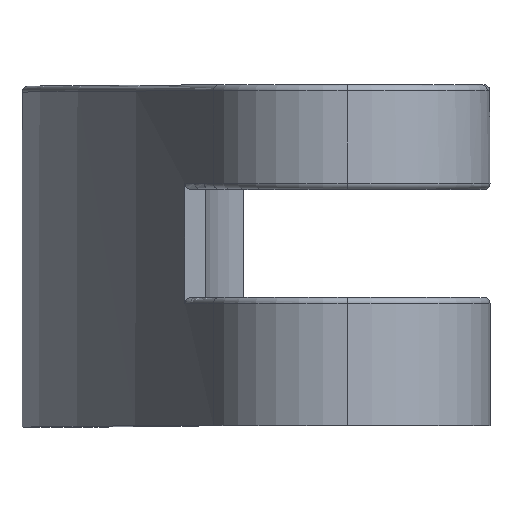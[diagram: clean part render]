
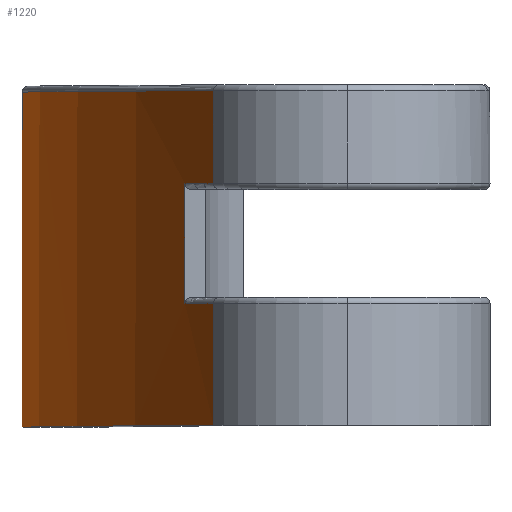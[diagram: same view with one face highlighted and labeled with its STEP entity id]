
A CAD part, top view. The second image highlights one B-rep face of the part: STEP entity #1220.
In plain terms, the highlighted cylindrical face has radius 180.483 mm (diameter 360.965 mm), a partial arc.
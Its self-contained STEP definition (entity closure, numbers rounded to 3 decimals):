
#23 = ORIENTED_EDGE ( 'NONE', *, *, #2267, .T. ) ;
#25 = DIRECTION ( 'NONE',  ( 0., 0., 1. ) ) ;
#28 = CIRCLE ( 'NONE', #1642, 180.483 ) ;
#90 = CARTESIAN_POINT ( 'NONE',  ( 169.67, 18.9, 51.202 ) ) ;
#130 = CIRCLE ( 'NONE', #591, 180.483 ) ;
#218 = ORIENTED_EDGE ( 'NONE', *, *, #2762, .T. ) ;
#219 = ORIENTED_EDGE ( 'NONE', *, *, #2981, .T. ) ;
#225 = CARTESIAN_POINT ( 'NONE',  ( 5.58, 9.9, 126.359 ) ) ;
#276 = VERTEX_POINT ( 'NONE', #3023 ) ;
#280 = CARTESIAN_POINT ( 'NONE',  ( -10.404, 18.905, 39.064 ) ) ;
#314 = ORIENTED_EDGE ( 'NONE', *, *, #1083, .T. ) ;
#316 = ORIENTED_EDGE ( 'NONE', *, *, #1071, .T. ) ;
#323 = CIRCLE ( 'NONE', #468, 180.483 ) ;
#340 = CIRCLE ( 'NONE', #2056, 180.483 ) ;
#357 = LINE ( 'NONE', #1776, #1922 ) ;
#375 = DIRECTION ( 'NONE',  ( 0., -1., 0. ) ) ;
#380 = VERTEX_POINT ( 'NONE', #2892 ) ;
#395 = EDGE_CURVE ( 'NONE', #1426, #1633, #1972, .T. ) ;
#398 = DIRECTION ( 'NONE',  ( 0., 1., 0. ) ) ;
#468 = AXIS2_PLACEMENT_3D ( 'NONE', #2551, #398, #1800 ) ;
#471 = CARTESIAN_POINT ( 'NONE',  ( 169.67, 20.1, 51.202 ) ) ;
#500 = LINE ( 'NONE', #1247, #1813 ) ;
#511 = CARTESIAN_POINT ( 'NONE',  ( 5.58, -0.5, 126.359 ) ) ;
#525 = VERTEX_POINT ( 'NONE', #511 ) ;
#527 = DIRECTION ( 'NONE',  ( 0., 1., 0. ) ) ;
#535 = ORIENTED_EDGE ( 'NONE', *, *, #674, .F. ) ;
#563 = AXIS2_PLACEMENT_3D ( 'NONE', #1868, #643, #1605 ) ;
#591 = AXIS2_PLACEMENT_3D ( 'NONE', #90, #1059, #824 ) ;
#606 = EDGE_CURVE ( 'NONE', #644, #525, #1523, .T. ) ;
#621 = VERTEX_POINT ( 'NONE', #1369 ) ;
#643 = DIRECTION ( 'NONE',  ( 0., 1., 0. ) ) ;
#644 = VERTEX_POINT ( 'NONE', #2547 ) ;
#652 = DIRECTION ( 'NONE',  ( 0., 0., 1. ) ) ;
#665 = DIRECTION ( 'NONE',  ( 0., 0., 1. ) ) ;
#674 = EDGE_CURVE ( 'NONE', #2632, #276, #500, .T. ) ;
#699 = CARTESIAN_POINT ( 'NONE',  ( 169.67, 1.5, 51.202 ) ) ;
#714 = DIRECTION ( 'NONE',  ( 0., -1., 0. ) ) ;
#804 = DIRECTION ( 'NONE',  ( 0., -1., 0. ) ) ;
#824 = DIRECTION ( 'NONE',  ( 0., 0., 1. ) ) ;
#849 = CARTESIAN_POINT ( 'NONE',  ( -9.893, 1.5, 33.005 ) ) ;
#903 = FACE_OUTER_BOUND ( 'NONE', #947, .T. ) ;
#911 = CIRCLE ( 'NONE', #2823, 180.483 ) ;
#931 = CARTESIAN_POINT ( 'NONE',  ( -10.404, 11.1, 39.064 ) ) ;
#944 = DIRECTION ( 'NONE',  ( 0., -1., 0. ) ) ;
#945 = ORIENTED_EDGE ( 'NONE', *, *, #606, .T. ) ;
#947 = EDGE_LOOP ( 'NONE', ( #23, #3118, #2841, #2101, #945, #316, #2026, #1456, #219, #1554, #314, #535, #218, #2310 ) ) ;
#981 = LINE ( 'NONE', #1218, #1594 ) ;
#1003 = CARTESIAN_POINT ( 'NONE',  ( 5.58, 28., 126.359 ) ) ;
#1051 = LINE ( 'NONE', #2693, #2529 ) ;
#1059 = DIRECTION ( 'NONE',  ( 0., -1., 0. ) ) ;
#1064 = CARTESIAN_POINT ( 'NONE',  ( 3.155, 20.1, 120.82 ) ) ;
#1071 = EDGE_CURVE ( 'NONE', #525, #1426, #357, .T. ) ;
#1083 = EDGE_CURVE ( 'NONE', #1778, #276, #911, .T. ) ;
#1111 = DIRECTION ( 'NONE',  ( 0., 1., 0. ) ) ;
#1127 = CARTESIAN_POINT ( 'NONE',  ( 3.155, 9.9, 120.82 ) ) ;
#1187 = CARTESIAN_POINT ( 'NONE',  ( -9.893, 11.1, 33.005 ) ) ;
#1218 = CARTESIAN_POINT ( 'NONE',  ( -10.404, 1.5, 39.064 ) ) ;
#1220 = ADVANCED_FACE ( 'NONE', ( #903 ), #1658, .T. ) ;
#1227 = VERTEX_POINT ( 'NONE', #1187 ) ;
#1247 = CARTESIAN_POINT ( 'NONE',  ( -10.428, 19.405, 39.43 ) ) ;
#1292 = CARTESIAN_POINT ( 'NONE',  ( -10.428, 18.905, 39.43 ) ) ;
#1369 = CARTESIAN_POINT ( 'NONE',  ( -10.404, 18.9, 39.064 ) ) ;
#1426 = VERTEX_POINT ( 'NONE', #225 ) ;
#1428 = CARTESIAN_POINT ( 'NONE',  ( 5.58, 20.1, 126.359 ) ) ;
#1456 = ORIENTED_EDGE ( 'NONE', *, *, #2203, .T. ) ;
#1470 = DIRECTION ( 'NONE',  ( 0., 0., -1. ) ) ;
#1523 = CIRCLE ( 'NONE', #563, 180.483 ) ;
#1553 = EDGE_CURVE ( 'NONE', #380, #1227, #2271, .T. ) ;
#1554 = ORIENTED_EDGE ( 'NONE', *, *, #1850, .T. ) ;
#1588 = DIRECTION ( 'NONE',  ( 0., 0., 1. ) ) ;
#1594 = VECTOR ( 'NONE', #2360, 1000. ) ;
#1599 = VECTOR ( 'NONE', #3094, 1000. ) ;
#1605 = DIRECTION ( 'NONE',  ( 0., 0., 1. ) ) ;
#1615 = DIRECTION ( 'NONE',  ( 0., 1., 0. ) ) ;
#1620 = VECTOR ( 'NONE', #804, 1000. ) ;
#1633 = VERTEX_POINT ( 'NONE', #1127 ) ;
#1642 = AXIS2_PLACEMENT_3D ( 'NONE', #471, #2172, #1470 ) ;
#1658 = CYLINDRICAL_SURFACE ( 'NONE', #2076, 180.483 ) ;
#1776 = CARTESIAN_POINT ( 'NONE',  ( 5.58, 1.5, 126.359 ) ) ;
#1778 = VERTEX_POINT ( 'NONE', #1003 ) ;
#1800 = DIRECTION ( 'NONE',  ( 0., 0., -1. ) ) ;
#1813 = VECTOR ( 'NONE', #2385, 1000. ) ;
#1850 = EDGE_CURVE ( 'NONE', #3047, #1778, #1051, .T. ) ;
#1868 = CARTESIAN_POINT ( 'NONE',  ( 169.67, -0.5, 51.202 ) ) ;
#1922 = VECTOR ( 'NONE', #1111, 1000. ) ;
#1939 = VERTEX_POINT ( 'NONE', #1064 ) ;
#1972 = CIRCLE ( 'NONE', #2730, 180.483 ) ;
#2026 = ORIENTED_EDGE ( 'NONE', *, *, #395, .T. ) ;
#2032 = DIRECTION ( 'NONE',  ( 0., 1., 0. ) ) ;
#2044 = EDGE_CURVE ( 'NONE', #1227, #3112, #323, .T. ) ;
#2056 = AXIS2_PLACEMENT_3D ( 'NONE', #3129, #944, #25 ) ;
#2076 = AXIS2_PLACEMENT_3D ( 'NONE', #699, #1615, #652 ) ;
#2101 = ORIENTED_EDGE ( 'NONE', *, *, #2946, .T. ) ;
#2121 = EDGE_CURVE ( 'NONE', #2294, #621, #981, .T. ) ;
#2172 = DIRECTION ( 'NONE',  ( 0., 1., 0. ) ) ;
#2203 = EDGE_CURVE ( 'NONE', #1633, #1939, #2689, .T. ) ;
#2232 = CARTESIAN_POINT ( 'NONE',  ( 3.155, 1.5, 120.82 ) ) ;
#2267 = EDGE_CURVE ( 'NONE', #621, #380, #130, .T. ) ;
#2271 = LINE ( 'NONE', #849, #1620 ) ;
#2294 = VERTEX_POINT ( 'NONE', #280 ) ;
#2310 = ORIENTED_EDGE ( 'NONE', *, *, #2121, .T. ) ;
#2336 = CARTESIAN_POINT ( 'NONE',  ( 169.67, 9.9, 51.202 ) ) ;
#2360 = DIRECTION ( 'NONE',  ( 0., -1., 0. ) ) ;
#2385 = DIRECTION ( 'NONE',  ( 0., 1., 0. ) ) ;
#2529 = VECTOR ( 'NONE', #2032, 1000. ) ;
#2547 = CARTESIAN_POINT ( 'NONE',  ( -10.404, -0.5, 39.064 ) ) ;
#2551 = CARTESIAN_POINT ( 'NONE',  ( 169.67, 11.1, 51.202 ) ) ;
#2554 = CARTESIAN_POINT ( 'NONE',  ( 169.67, 28., 51.202 ) ) ;
#2632 = VERTEX_POINT ( 'NONE', #1292 ) ;
#2663 = LINE ( 'NONE', #2900, #1599 ) ;
#2689 = LINE ( 'NONE', #2232, #2843 ) ;
#2693 = CARTESIAN_POINT ( 'NONE',  ( 5.58, 1.5, 126.359 ) ) ;
#2730 = AXIS2_PLACEMENT_3D ( 'NONE', #2336, #714, #665 ) ;
#2762 = EDGE_CURVE ( 'NONE', #2632, #2294, #340, .T. ) ;
#2823 = AXIS2_PLACEMENT_3D ( 'NONE', #2554, #375, #1588 ) ;
#2841 = ORIENTED_EDGE ( 'NONE', *, *, #2044, .T. ) ;
#2843 = VECTOR ( 'NONE', #527, 1000. ) ;
#2892 = CARTESIAN_POINT ( 'NONE',  ( -9.893, 18.9, 33.005 ) ) ;
#2900 = CARTESIAN_POINT ( 'NONE',  ( -10.404, 13.998, 39.064 ) ) ;
#2946 = EDGE_CURVE ( 'NONE', #3112, #644, #2663, .T. ) ;
#2981 = EDGE_CURVE ( 'NONE', #1939, #3047, #28, .T. ) ;
#3023 = CARTESIAN_POINT ( 'NONE',  ( -10.428, 28., 39.43 ) ) ;
#3047 = VERTEX_POINT ( 'NONE', #1428 ) ;
#3094 = DIRECTION ( 'NONE',  ( 0., -1., 0. ) ) ;
#3112 = VERTEX_POINT ( 'NONE', #931 ) ;
#3118 = ORIENTED_EDGE ( 'NONE', *, *, #1553, .T. ) ;
#3129 = CARTESIAN_POINT ( 'NONE',  ( 169.67, 18.905, 51.202 ) ) ;
